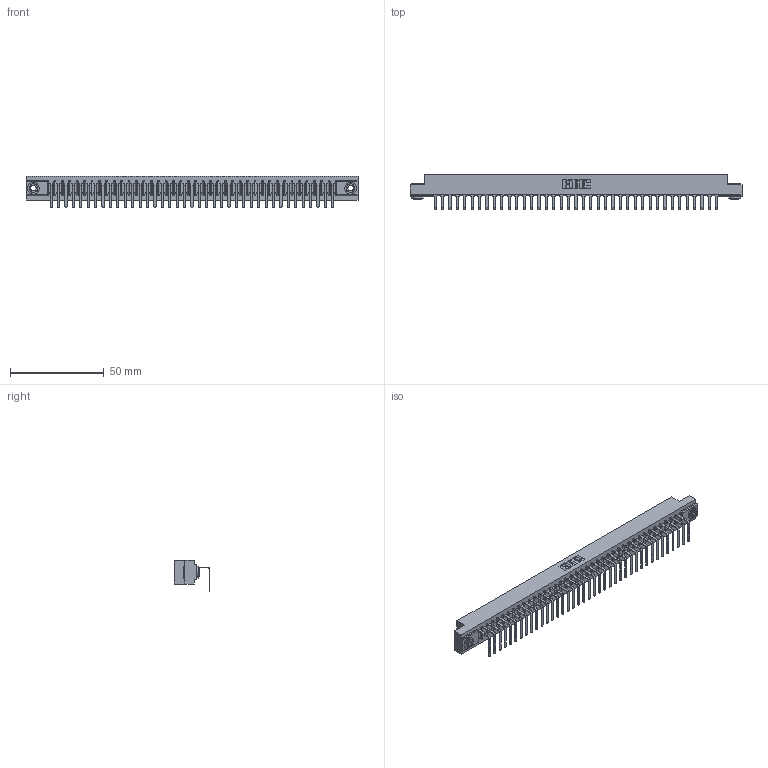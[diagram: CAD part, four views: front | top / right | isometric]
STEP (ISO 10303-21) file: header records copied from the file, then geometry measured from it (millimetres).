
FILE_DESCRIPTION (( 'STEP AP203' ), '1' );
FILE_NAME ('307-039-558-103.STEP', '2019-09-05T14:53:40', ( '' ), ( '' ), 'SwSTEP 2.0', 'SolidWorks 2016', '' );
FILE_SCHEMA (( 'CONFIG_CONTROL_DESIGN' ));
Length unit declared in the file: inch
Products named in the file (4): 307 Part_.156 Dia Mounting Holes; 345-250-002_345-250-002-102; 307-290-001_558 - 2 (Single); 307-039-558-103
Assembly tree (42 placements, depth 2):
  307-039-558-103
    307 Part_.156 Dia Mounting Holes
    307-290-001_558 - 2 (Single)  x39
    345-250-002_345-250-002-102  x2
Bounding box: 177.55 x 18.96 x 16.8 mm (x, y, z)
Volume: 18592.5 mm3; surface area: 21053 mm2
Topology: 42 solids, 42 shells, 2550 faces, 7221 edges, 4650 vertices
Faces by surface type: plane 1615, cylinder 847, sphere 80, cone 8
Entity records: 34973 total; most frequent: CARTESIAN_POINT 5869, ORIENTED_EDGE 5846, DIRECTION 5725, EDGE_CURVE 2923, VECTOR 2233, LINE 2233, VERTEX_POINT 1890, AXIS2_PLACEMENT_3D 1746
